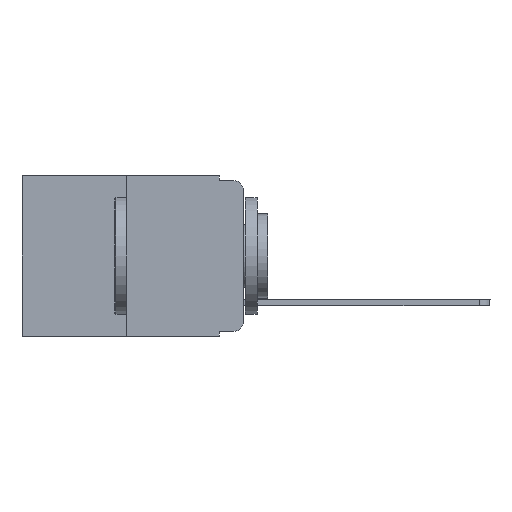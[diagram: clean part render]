
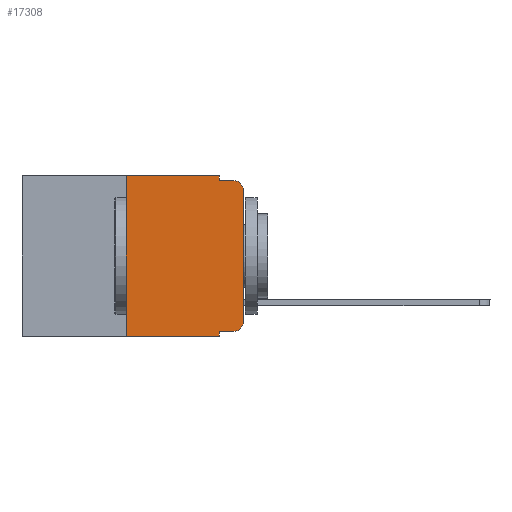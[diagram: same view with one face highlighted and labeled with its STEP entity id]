
A CAD part, left-side view. The second image highlights one B-rep face of the part: STEP entity #17308.
In plain terms, the highlighted planar face has unit normal (-1, 0, 0).
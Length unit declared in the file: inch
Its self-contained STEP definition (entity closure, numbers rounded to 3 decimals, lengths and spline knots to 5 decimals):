
#129 = LINE ( 'NONE', #12802, #10417 ) ;
#248 = ORIENTED_EDGE ( 'NONE', *, *, #8914, .F. ) ;
#703 = VERTEX_POINT ( 'NONE', #3915 ) ;
#750 = LINE ( 'NONE', #2381, #17931 ) ;
#893 = EDGE_CURVE ( 'NONE', #14288, #8193, #6653, .T. ) ;
#1360 = CARTESIAN_POINT ( 'NONE',  ( 0., 0.25, 0. ) ) ;
#1641 = ORIENTED_EDGE ( 'NONE', *, *, #893, .T. ) ;
#1700 = DIRECTION ( 'NONE',  ( 0., 0., -1. ) ) ;
#2083 = LINE ( 'NONE', #13027, #17850 ) ;
#2184 = CARTESIAN_POINT ( 'NONE',  ( 0., 0.473, -0.343 ) ) ;
#2381 = CARTESIAN_POINT ( 'NONE',  ( 0., 0.25, 0. ) ) ;
#2480 = DIRECTION ( 'NONE',  ( 0., 0., -1. ) ) ;
#2679 = DIRECTION ( 'NONE',  ( -1., 0., 0. ) ) ;
#2865 = VERTEX_POINT ( 'NONE', #10958 ) ;
#2932 = VECTOR ( 'NONE', #11480, 39.37008 ) ;
#2933 = DIRECTION ( 'NONE',  ( 0., 0., -1. ) ) ;
#3219 = AXIS2_PLACEMENT_3D ( 'NONE', #12884, #19101, #5129 ) ;
#3424 = DIRECTION ( 'NONE',  ( -1., 0., 0. ) ) ;
#3670 = CARTESIAN_POINT ( 'NONE',  ( 0., 0., -0.313 ) ) ;
#3708 = EDGE_CURVE ( 'NONE', #2865, #14288, #15285, .T. ) ;
#3807 = LINE ( 'NONE', #8594, #8423 ) ;
#3915 = CARTESIAN_POINT ( 'NONE',  ( 0., 0.051, 0. ) ) ;
#4335 = EDGE_CURVE ( 'NONE', #703, #8105, #3807, .T. ) ;
#4503 = EDGE_CURVE ( 'NONE', #8193, #18832, #5204, .T. ) ;
#4649 = CARTESIAN_POINT ( 'NONE',  ( 0., 0.051, 0. ) ) ;
#4936 = DIRECTION ( 'NONE',  ( 0., -1., 0. ) ) ;
#5129 = DIRECTION ( 'NONE',  ( 0., 0., -1. ) ) ;
#5204 = CIRCLE ( 'NONE', #6823, 0.02 ) ;
#5618 = EDGE_CURVE ( 'NONE', #18003, #14557, #6792, .T. ) ;
#5698 = EDGE_CURVE ( 'NONE', #18003, #10439, #750, .T. ) ;
#6653 = LINE ( 'NONE', #9602, #10252 ) ;
#6655 = PLANE ( 'NONE',  #3219 ) ;
#6693 = EDGE_CURVE ( 'NONE', #8105, #18832, #2083, .T. ) ;
#6792 = LINE ( 'NONE', #2184, #2932 ) ;
#6823 = AXIS2_PLACEMENT_3D ( 'NONE', #16674, #2679, #2480 ) ;
#7489 = LINE ( 'NONE', #16466, #17878 ) ;
#8105 = VERTEX_POINT ( 'NONE', #10852 ) ;
#8186 = FACE_OUTER_BOUND ( 'NONE', #9457, .T. ) ;
#8193 = VERTEX_POINT ( 'NONE', #19936 ) ;
#8329 = EDGE_CURVE ( 'NONE', #18531, #2865, #129, .T. ) ;
#8393 = ORIENTED_EDGE ( 'NONE', *, *, #4503, .T. ) ;
#8423 = VECTOR ( 'NONE', #10138, 39.37008 ) ;
#8594 = CARTESIAN_POINT ( 'NONE',  ( 0., 0.051, 0. ) ) ;
#8600 = DIRECTION ( 'NONE',  ( 0., 0., 1. ) ) ;
#8914 = EDGE_CURVE ( 'NONE', #18531, #14557, #11101, .T. ) ;
#9042 = ORIENTED_EDGE ( 'NONE', *, *, #5698, .F. ) ;
#9457 = EDGE_LOOP ( 'NONE', ( #1641, #8393, #10174, #18651, #16380, #9042, #15723, #248, #11726, #16213 ) ) ;
#9602 = CARTESIAN_POINT ( 'NONE',  ( 0., 0., 0. ) ) ;
#10138 = DIRECTION ( 'NONE',  ( 0., 0., -1. ) ) ;
#10174 = ORIENTED_EDGE ( 'NONE', *, *, #6693, .F. ) ;
#10252 = VECTOR ( 'NONE', #17278, 39.37008 ) ;
#10417 = VECTOR ( 'NONE', #4936, 39.37008 ) ;
#10439 = VERTEX_POINT ( 'NONE', #1360 ) ;
#10852 = CARTESIAN_POINT ( 'NONE',  ( 0., 0.051, -0.01 ) ) ;
#10957 = CARTESIAN_POINT ( 'NONE',  ( 0., 0.02, -0.01 ) ) ;
#10958 = CARTESIAN_POINT ( 'NONE',  ( 0., 0.02, -0.333 ) ) ;
#11101 = LINE ( 'NONE', #4649, #16846 ) ;
#11276 = DIRECTION ( 'NONE',  ( 0., -1., 0. ) ) ;
#11348 = AXIS2_PLACEMENT_3D ( 'NONE', #16009, #3424, #1700 ) ;
#11480 = DIRECTION ( 'NONE',  ( 0., -1., 0. ) ) ;
#11586 = CARTESIAN_POINT ( 'NONE',  ( 0., 0.051, -0.333 ) ) ;
#11726 = ORIENTED_EDGE ( 'NONE', *, *, #8329, .T. ) ;
#12802 = CARTESIAN_POINT ( 'NONE',  ( 0., 0.051, -0.333 ) ) ;
#12884 = CARTESIAN_POINT ( 'NONE',  ( 0., 0.473, 0. ) ) ;
#13027 = CARTESIAN_POINT ( 'NONE',  ( 0., 0.051, -0.01 ) ) ;
#14288 = VERTEX_POINT ( 'NONE', #3670 ) ;
#14557 = VERTEX_POINT ( 'NONE', #17554 ) ;
#15285 = CIRCLE ( 'NONE', #11348, 0.02 ) ;
#15723 = ORIENTED_EDGE ( 'NONE', *, *, #5618, .T. ) ;
#16009 = CARTESIAN_POINT ( 'NONE',  ( 0., 0.02, -0.313 ) ) ;
#16213 = ORIENTED_EDGE ( 'NONE', *, *, #3708, .T. ) ;
#16380 = ORIENTED_EDGE ( 'NONE', *, *, #16978, .F. ) ;
#16466 = CARTESIAN_POINT ( 'NONE',  ( 0., 0.473, 0. ) ) ;
#16674 = CARTESIAN_POINT ( 'NONE',  ( 0., 0.02, -0.03 ) ) ;
#16846 = VECTOR ( 'NONE', #2933, 39.37008 ) ;
#16978 = EDGE_CURVE ( 'NONE', #10439, #703, #7489, .T. ) ;
#17269 = CARTESIAN_POINT ( 'NONE',  ( 0., 0.25, -0.343 ) ) ;
#17278 = DIRECTION ( 'NONE',  ( 0., 0., 1. ) ) ;
#17308 = ADVANCED_FACE ( 'NONE', ( #8186 ), #6655, .F. ) ;
#17554 = CARTESIAN_POINT ( 'NONE',  ( 0., 0.051, -0.343 ) ) ;
#17850 = VECTOR ( 'NONE', #11276, 39.37008 ) ;
#17878 = VECTOR ( 'NONE', #19924, 39.37008 ) ;
#17931 = VECTOR ( 'NONE', #8600, 39.37008 ) ;
#18003 = VERTEX_POINT ( 'NONE', #17269 ) ;
#18531 = VERTEX_POINT ( 'NONE', #11586 ) ;
#18651 = ORIENTED_EDGE ( 'NONE', *, *, #4335, .F. ) ;
#18832 = VERTEX_POINT ( 'NONE', #10957 ) ;
#19101 = DIRECTION ( 'NONE',  ( 1., 0., 0. ) ) ;
#19924 = DIRECTION ( 'NONE',  ( 0., -1., 0. ) ) ;
#19936 = CARTESIAN_POINT ( 'NONE',  ( 0., 0., -0.03 ) ) ;
